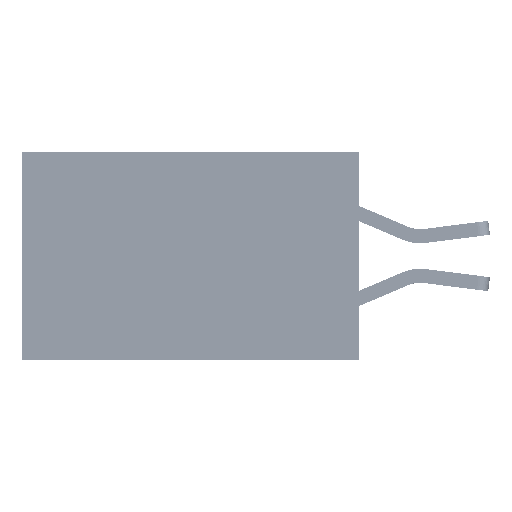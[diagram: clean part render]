
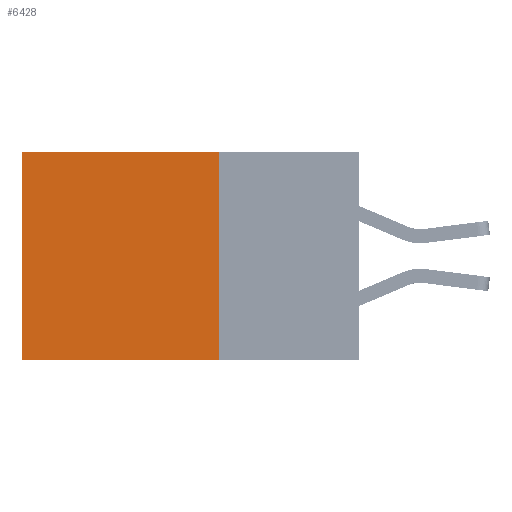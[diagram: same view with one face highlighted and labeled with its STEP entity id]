
A CAD part, left-side view. The second image highlights one B-rep face of the part: STEP entity #6428.
In plain terms, the highlighted planar face has unit normal (-1, 0, 0).
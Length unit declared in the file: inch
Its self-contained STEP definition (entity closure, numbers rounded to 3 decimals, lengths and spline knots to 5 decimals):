
#642 = VERTEX_POINT ( 'NONE', #18787 ) ;
#2411 = CARTESIAN_POINT ( 'NONE',  ( 0.2875, 0.6, -0.37 ) ) ;
#2544 = EDGE_CURVE ( 'NONE', #33501, #12965, #21026, .T. ) ;
#4446 = CARTESIAN_POINT ( 'NONE',  ( 0.2875, 0.25, 0. ) ) ;
#4990 = CARTESIAN_POINT ( 'NONE',  ( 0.2875, 0.25, -0.37 ) ) ;
#5980 = CARTESIAN_POINT ( 'NONE',  ( 0.2875, 0.25, 0. ) ) ;
#6428 = ADVANCED_FACE ( 'NONE', ( #19593 ), #45227, .F. ) ;
#7944 = VECTOR ( 'NONE', #8834, 39.37008 ) ;
#8834 = DIRECTION ( 'NONE',  ( 0., 1., 0. ) ) ;
#9573 = DIRECTION ( 'NONE',  ( 1., 0., 0. ) ) ;
#9844 = VECTOR ( 'NONE', #30970, 39.37008 ) ;
#11730 = VECTOR ( 'NONE', #22096, 39.37008 ) ;
#12849 = DIRECTION ( 'NONE',  ( 0., 0., -1. ) ) ;
#12965 = VERTEX_POINT ( 'NONE', #2411 ) ;
#13552 = CARTESIAN_POINT ( 'NONE',  ( 0.2875, 0.25, -0.37 ) ) ;
#14732 = EDGE_CURVE ( 'NONE', #642, #33501, #19102, .T. ) ;
#14772 = AXIS2_PLACEMENT_3D ( 'NONE', #5980, #9573, #12849 ) ;
#15525 = ORIENTED_EDGE ( 'NONE', *, *, #2544, .T. ) ;
#16456 = CARTESIAN_POINT ( 'NONE',  ( 0.2875, 0.25, 0. ) ) ;
#18787 = CARTESIAN_POINT ( 'NONE',  ( 0.2875, 0.25, 0. ) ) ;
#19102 = LINE ( 'NONE', #16456, #7944 ) ;
#19593 = FACE_OUTER_BOUND ( 'NONE', #23597, .T. ) ;
#21026 = LINE ( 'NONE', #23451, #9844 ) ;
#22096 = DIRECTION ( 'NONE',  ( 0., 0., -1. ) ) ;
#22406 = VECTOR ( 'NONE', #27209, 39.37008 ) ;
#23451 = CARTESIAN_POINT ( 'NONE',  ( 0.2875, 0.6, 0. ) ) ;
#23597 = EDGE_LOOP ( 'NONE', ( #15525, #33378, #31829, #38317 ) ) ;
#27209 = DIRECTION ( 'NONE',  ( 0., 1., 0. ) ) ;
#27789 = EDGE_CURVE ( 'NONE', #642, #28098, #44175, .T. ) ;
#28098 = VERTEX_POINT ( 'NONE', #13552 ) ;
#30970 = DIRECTION ( 'NONE',  ( 0., 0., -1. ) ) ;
#31829 = ORIENTED_EDGE ( 'NONE', *, *, #27789, .F. ) ;
#33378 = ORIENTED_EDGE ( 'NONE', *, *, #35960, .F. ) ;
#33501 = VERTEX_POINT ( 'NONE', #45710 ) ;
#35960 = EDGE_CURVE ( 'NONE', #28098, #12965, #42559, .T. ) ;
#38317 = ORIENTED_EDGE ( 'NONE', *, *, #14732, .T. ) ;
#42559 = LINE ( 'NONE', #4990, #22406 ) ;
#44175 = LINE ( 'NONE', #4446, #11730 ) ;
#45227 = PLANE ( 'NONE',  #14772 ) ;
#45710 = CARTESIAN_POINT ( 'NONE',  ( 0.2875, 0.6, 0. ) ) ;
